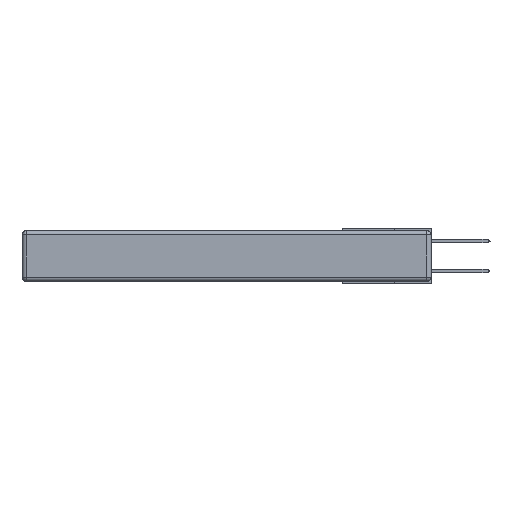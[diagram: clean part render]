
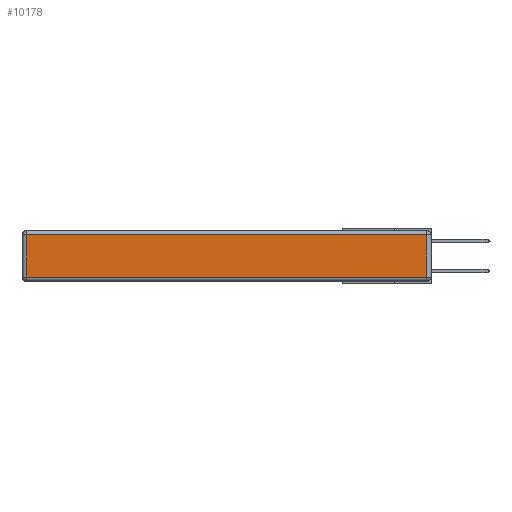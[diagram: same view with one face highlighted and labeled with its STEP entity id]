
A CAD part, left-side view. The second image highlights one B-rep face of the part: STEP entity #10178.
In plain terms, the highlighted planar face has unit normal (-1, 0, 0).
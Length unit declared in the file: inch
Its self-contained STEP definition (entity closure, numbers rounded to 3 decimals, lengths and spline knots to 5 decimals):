
#98 = DIRECTION ( 'NONE',  ( 0., 1., 0. ) ) ;
#1688 = CARTESIAN_POINT ( 'NONE',  ( 0., 0., -0.313 ) ) ;
#1885 = ORIENTED_EDGE ( 'NONE', *, *, #4337, .T. ) ;
#2245 = EDGE_CURVE ( 'NONE', #5884, #12873, #2762, .T. ) ;
#2762 = LINE ( 'NONE', #28156, #8865 ) ;
#4293 = CARTESIAN_POINT ( 'NONE',  ( 0., 0.03, -0.313 ) ) ;
#4337 = EDGE_CURVE ( 'NONE', #12873, #18998, #18753, .T. ) ;
#5573 = ORIENTED_EDGE ( 'NONE', *, *, #2245, .T. ) ;
#5715 = FACE_OUTER_BOUND ( 'NONE', #26164, .T. ) ;
#5884 = VERTEX_POINT ( 'NONE', #13008 ) ;
#6384 = VECTOR ( 'NONE', #98, 39.37008 ) ;
#6854 = ORIENTED_EDGE ( 'NONE', *, *, #30967, .T. ) ;
#8865 = VECTOR ( 'NONE', #18212, 39.37008 ) ;
#9169 = AXIS2_PLACEMENT_3D ( 'NONE', #22282, #20245, #22490 ) ;
#10178 = ADVANCED_FACE ( 'NONE', ( #5715 ), #17395, .T. ) ;
#12216 = VERTEX_POINT ( 'NONE', #18293 ) ;
#12873 = VERTEX_POINT ( 'NONE', #29304 ) ;
#13008 = CARTESIAN_POINT ( 'NONE',  ( 0., 2.72, -0.03 ) ) ;
#13963 = DIRECTION ( 'NONE',  ( 0., -1., 0. ) ) ;
#17395 = PLANE ( 'NONE',  #9169 ) ;
#18212 = DIRECTION ( 'NONE',  ( 0., 0., -1. ) ) ;
#18293 = CARTESIAN_POINT ( 'NONE',  ( 0., 0.03, -0.03 ) ) ;
#18753 = LINE ( 'NONE', #1688, #27102 ) ;
#18998 = VERTEX_POINT ( 'NONE', #4293 ) ;
#19688 = LINE ( 'NONE', #29323, #6384 ) ;
#20245 = DIRECTION ( 'NONE',  ( -1., 0., 0. ) ) ;
#21107 = VECTOR ( 'NONE', #27577, 39.37008 ) ;
#22282 = CARTESIAN_POINT ( 'NONE',  ( 0., 0., -0.343 ) ) ;
#22490 = DIRECTION ( 'NONE',  ( 0., 0., 1. ) ) ;
#25140 = CARTESIAN_POINT ( 'NONE',  ( 0., 0.03, -0.343 ) ) ;
#26164 = EDGE_LOOP ( 'NONE', ( #1885, #6854, #29657, #5573 ) ) ;
#27102 = VECTOR ( 'NONE', #13963, 39.37008 ) ;
#27577 = DIRECTION ( 'NONE',  ( 0., 0., 1. ) ) ;
#28156 = CARTESIAN_POINT ( 'NONE',  ( 0., 2.72, -0.343 ) ) ;
#29304 = CARTESIAN_POINT ( 'NONE',  ( 0., 2.72, -0.313 ) ) ;
#29323 = CARTESIAN_POINT ( 'NONE',  ( 0., 2.75, -0.03 ) ) ;
#29428 = EDGE_CURVE ( 'NONE', #12216, #5884, #19688, .T. ) ;
#29657 = ORIENTED_EDGE ( 'NONE', *, *, #29428, .T. ) ;
#30212 = LINE ( 'NONE', #25140, #21107 ) ;
#30967 = EDGE_CURVE ( 'NONE', #18998, #12216, #30212, .T. ) ;
